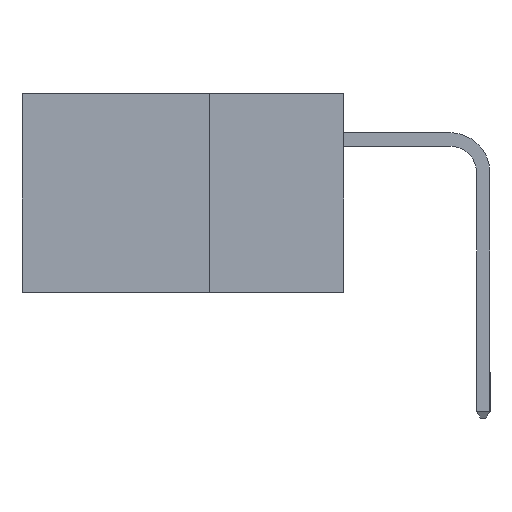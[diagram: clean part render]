
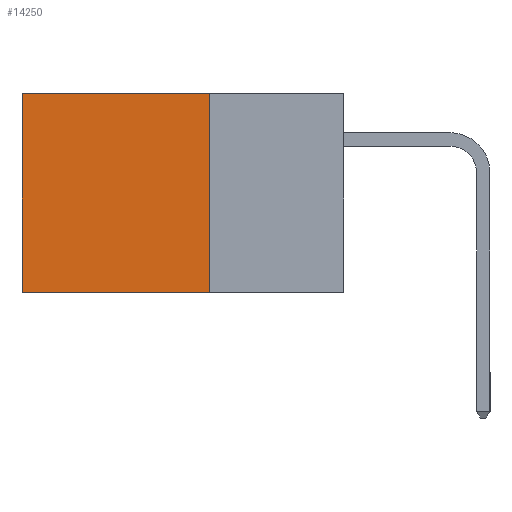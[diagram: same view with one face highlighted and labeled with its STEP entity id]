
A CAD part, left-side view. The second image highlights one B-rep face of the part: STEP entity #14250.
In plain terms, the highlighted planar face has unit normal (-1, 0, 0).
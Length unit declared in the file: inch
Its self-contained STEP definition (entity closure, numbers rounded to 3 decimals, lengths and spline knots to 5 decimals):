
#257 = EDGE_CURVE ( 'NONE', #16886, #6724, #9337, .T. ) ;
#1237 = LINE ( 'NONE', #11804, #15167 ) ;
#1708 = CARTESIAN_POINT ( 'NONE',  ( 0.298, 0.25, 0. ) ) ;
#2514 = VECTOR ( 'NONE', #19871, 39.37008 ) ;
#2629 = CARTESIAN_POINT ( 'NONE',  ( 0.298, 0.25, -0.37 ) ) ;
#6444 = CARTESIAN_POINT ( 'NONE',  ( 0.298, 0.6, 0. ) ) ;
#6724 = VERTEX_POINT ( 'NONE', #21318 ) ;
#8690 = VERTEX_POINT ( 'NONE', #2629 ) ;
#8885 = CARTESIAN_POINT ( 'NONE',  ( 0.298, 0.25, 0. ) ) ;
#9147 = DIRECTION ( 'NONE',  ( 0., 1., 0. ) ) ;
#9171 = VERTEX_POINT ( 'NONE', #15139 ) ;
#9337 = LINE ( 'NONE', #16005, #2514 ) ;
#9407 = PLANE ( 'NONE',  #12267 ) ;
#9919 = EDGE_CURVE ( 'NONE', #9171, #16886, #15214, .T. ) ;
#10018 = VECTOR ( 'NONE', #9147, 39.37008 ) ;
#10704 = EDGE_CURVE ( 'NONE', #9171, #8690, #1237, .T. ) ;
#11804 = CARTESIAN_POINT ( 'NONE',  ( 0.298, 0.25, 0. ) ) ;
#12267 = AXIS2_PLACEMENT_3D ( 'NONE', #1708, #18822, #20723 ) ;
#14217 = EDGE_LOOP ( 'NONE', ( #21912, #20099, #17217, #23902 ) ) ;
#14250 = ADVANCED_FACE ( 'NONE', ( #17305 ), #9407, .F. ) ;
#15139 = CARTESIAN_POINT ( 'NONE',  ( 0.298, 0.25, 0. ) ) ;
#15167 = VECTOR ( 'NONE', #23209, 39.37008 ) ;
#15214 = LINE ( 'NONE', #8885, #19629 ) ;
#15632 = LINE ( 'NONE', #16997, #10018 ) ;
#16005 = CARTESIAN_POINT ( 'NONE',  ( 0.298, 0.6, 0. ) ) ;
#16886 = VERTEX_POINT ( 'NONE', #6444 ) ;
#16997 = CARTESIAN_POINT ( 'NONE',  ( 0.298, 0.25, -0.37 ) ) ;
#17217 = ORIENTED_EDGE ( 'NONE', *, *, #10704, .F. ) ;
#17305 = FACE_OUTER_BOUND ( 'NONE', #14217, .T. ) ;
#18822 = DIRECTION ( 'NONE',  ( 1., 0., 0. ) ) ;
#19113 = EDGE_CURVE ( 'NONE', #8690, #6724, #15632, .T. ) ;
#19629 = VECTOR ( 'NONE', #22109, 39.37008 ) ;
#19871 = DIRECTION ( 'NONE',  ( 0., 0., -1. ) ) ;
#20099 = ORIENTED_EDGE ( 'NONE', *, *, #19113, .F. ) ;
#20723 = DIRECTION ( 'NONE',  ( 0., 0., -1. ) ) ;
#21318 = CARTESIAN_POINT ( 'NONE',  ( 0.298, 0.6, -0.37 ) ) ;
#21912 = ORIENTED_EDGE ( 'NONE', *, *, #257, .T. ) ;
#22109 = DIRECTION ( 'NONE',  ( 0., 1., 0. ) ) ;
#23209 = DIRECTION ( 'NONE',  ( 0., 0., -1. ) ) ;
#23902 = ORIENTED_EDGE ( 'NONE', *, *, #9919, .T. ) ;
